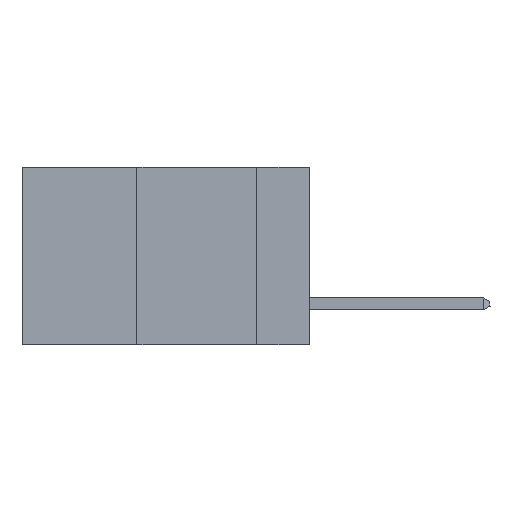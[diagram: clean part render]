
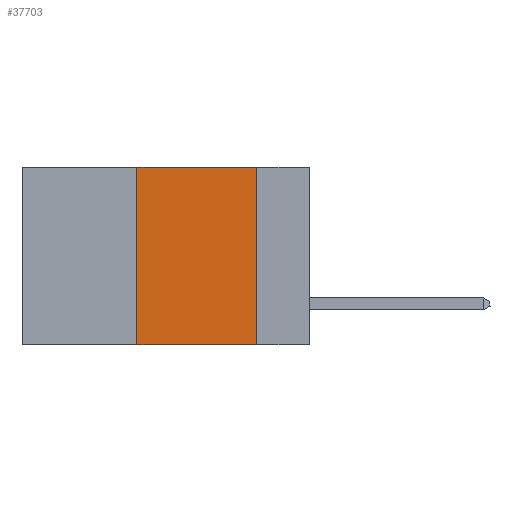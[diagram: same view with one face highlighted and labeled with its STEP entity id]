
A CAD part, left-side view. The second image highlights one B-rep face of the part: STEP entity #37703.
In plain terms, the highlighted planar face has unit normal (-1, 0, 0).
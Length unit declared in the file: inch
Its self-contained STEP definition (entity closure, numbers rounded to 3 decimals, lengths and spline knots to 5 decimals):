
#436 = VERTEX_POINT ( 'NONE', #8340 ) ;
#556 = VERTEX_POINT ( 'NONE', #16076 ) ;
#1048 = DIRECTION ( 'NONE',  ( 0., 0., -1. ) ) ;
#1265 = EDGE_CURVE ( 'NONE', #21768, #556, #21857, .T. ) ;
#2179 = CARTESIAN_POINT ( 'NONE',  ( 0., 0.36, 0. ) ) ;
#2454 = DIRECTION ( 'NONE',  ( 0., 0., 1. ) ) ;
#3132 = PLANE ( 'NONE',  #20463 ) ;
#5423 = VERTEX_POINT ( 'NONE', #9377 ) ;
#6400 = CARTESIAN_POINT ( 'NONE',  ( 0., 0.6, 0. ) ) ;
#6658 = LINE ( 'NONE', #11042, #30626 ) ;
#8340 = CARTESIAN_POINT ( 'NONE',  ( 0., 0.11, 0. ) ) ;
#9352 = DIRECTION ( 'NONE',  ( 0., -1., 0. ) ) ;
#9377 = CARTESIAN_POINT ( 'NONE',  ( 0., 0.36, 0. ) ) ;
#11042 = CARTESIAN_POINT ( 'NONE',  ( 0., 0.11, 0. ) ) ;
#11517 = FACE_OUTER_BOUND ( 'NONE', #15219, .T. ) ;
#12843 = VECTOR ( 'NONE', #2454, 39.37008 ) ;
#14581 = EDGE_CURVE ( 'NONE', #436, #556, #6658, .T. ) ;
#15219 = EDGE_LOOP ( 'NONE', ( #35215, #34043, #37775, #24824 ) ) ;
#16076 = CARTESIAN_POINT ( 'NONE',  ( 0., 0.11, -0.37 ) ) ;
#16813 = VECTOR ( 'NONE', #9352, 39.37008 ) ;
#19447 = CARTESIAN_POINT ( 'NONE',  ( 0., 0.6, -0.37 ) ) ;
#20463 = AXIS2_PLACEMENT_3D ( 'NONE', #6400, #32490, #28920 ) ;
#21768 = VERTEX_POINT ( 'NONE', #32581 ) ;
#21857 = LINE ( 'NONE', #19447, #16813 ) ;
#23501 = LINE ( 'NONE', #2179, #12843 ) ;
#24824 = ORIENTED_EDGE ( 'NONE', *, *, #1265, .T. ) ;
#28920 = DIRECTION ( 'NONE',  ( 0., 0., -1. ) ) ;
#30626 = VECTOR ( 'NONE', #1048, 39.37008 ) ;
#32490 = DIRECTION ( 'NONE',  ( 1., 0., 0. ) ) ;
#32581 = CARTESIAN_POINT ( 'NONE',  ( 0., 0.36, -0.37 ) ) ;
#32588 = VECTOR ( 'NONE', #33612, 39.37008 ) ;
#33612 = DIRECTION ( 'NONE',  ( 0., -1., 0. ) ) ;
#34043 = ORIENTED_EDGE ( 'NONE', *, *, #41145, .F. ) ;
#35215 = ORIENTED_EDGE ( 'NONE', *, *, #14581, .F. ) ;
#37286 = CARTESIAN_POINT ( 'NONE',  ( 0., 0.6, 0. ) ) ;
#37703 = ADVANCED_FACE ( 'NONE', ( #11517 ), #3132, .F. ) ;
#37775 = ORIENTED_EDGE ( 'NONE', *, *, #39945, .F. ) ;
#39945 = EDGE_CURVE ( 'NONE', #21768, #5423, #23501, .T. ) ;
#41145 = EDGE_CURVE ( 'NONE', #5423, #436, #41250, .T. ) ;
#41250 = LINE ( 'NONE', #37286, #32588 ) ;
